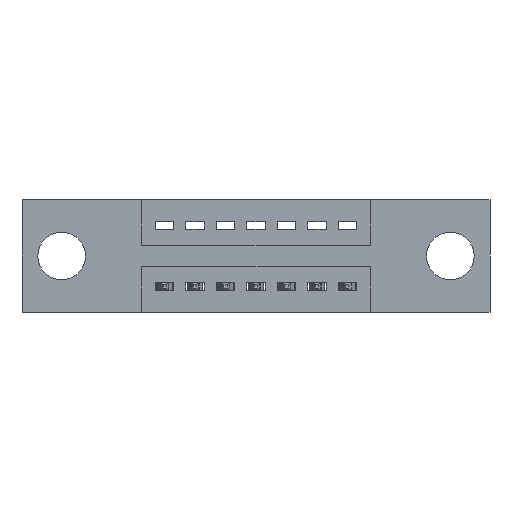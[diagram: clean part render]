
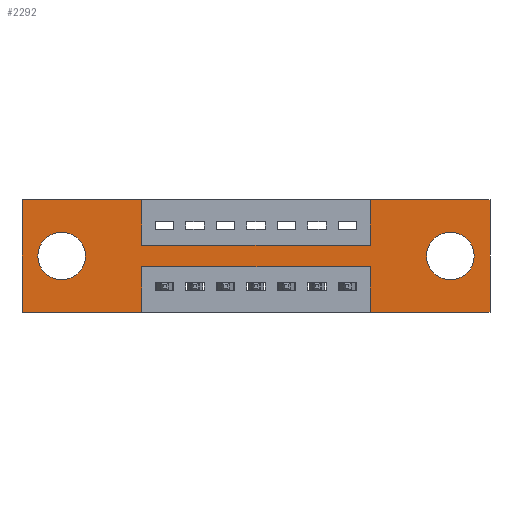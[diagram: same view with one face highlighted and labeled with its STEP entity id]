
A CAD part, front view. The second image highlights one B-rep face of the part: STEP entity #2292.
In plain terms, the highlighted planar face has unit normal (0, -1, 0).
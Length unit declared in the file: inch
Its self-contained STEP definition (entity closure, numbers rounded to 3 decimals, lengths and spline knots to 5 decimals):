
#102 = VERTEX_POINT ( 'NONE', #5162 ) ;
#122 = VERTEX_POINT ( 'NONE', #610 ) ;
#315 = CARTESIAN_POINT ( 'NONE',  ( 1.535, 0., -0.37 ) ) ;
#375 = DIRECTION ( 'NONE',  ( 0., 0., -1. ) ) ;
#422 = PLANE ( 'NONE',  #8379 ) ;
#440 = CARTESIAN_POINT ( 'NONE',  ( 0., 0., -0.37 ) ) ;
#477 = EDGE_CURVE ( 'NONE', #102, #6593, #5903, .T. ) ;
#610 = CARTESIAN_POINT ( 'NONE',  ( 1.405, 0., -0.107 ) ) ;
#1082 = DIRECTION ( 'NONE',  ( 1., 0., 0. ) ) ;
#1196 = DIRECTION ( 'NONE',  ( 0., 1., 0. ) ) ;
#1206 = DIRECTION ( 'NONE',  ( 0., 1., 0. ) ) ;
#1230 = VERTEX_POINT ( 'NONE', #7979 ) ;
#1262 = CARTESIAN_POINT ( 'NONE',  ( 0.3925, 0., -0.22 ) ) ;
#1273 = EDGE_CURVE ( 'NONE', #1230, #5263, #3168, .T. ) ;
#1364 = AXIS2_PLACEMENT_3D ( 'NONE', #6124, #1196, #6824 ) ;
#1372 = VERTEX_POINT ( 'NONE', #6577 ) ;
#1418 = EDGE_CURVE ( 'NONE', #3065, #1230, #2314, .T. ) ;
#1561 = VECTOR ( 'NONE', #375, 39.37008 ) ;
#1761 = EDGE_CURVE ( 'NONE', #5263, #1372, #2443, .T. ) ;
#1782 = EDGE_LOOP ( 'NONE', ( #3721, #3647 ) ) ;
#1783 = EDGE_LOOP ( 'NONE', ( #6504, #3783, #6387, #6543, #3159, #2726, #2746, #2822, #3049, #3062, #4244, #8692 ) ) ;
#1790 = DIRECTION ( 'NONE',  ( 0., 0., 1. ) ) ;
#1834 = CARTESIAN_POINT ( 'NONE',  ( 1.1425, 0., 0. ) ) ;
#1880 = LINE ( 'NONE', #9685, #5927 ) ;
#1946 = CARTESIAN_POINT ( 'NONE',  ( 0.3925, 0., 0. ) ) ;
#2059 = DIRECTION ( 'NONE',  ( 0., 1., 0. ) ) ;
#2099 = CARTESIAN_POINT ( 'NONE',  ( 1.535, 0., 0. ) ) ;
#2210 = VECTOR ( 'NONE', #1790, 39.37008 ) ;
#2235 = CARTESIAN_POINT ( 'NONE',  ( 0.3925, 0., -0.15 ) ) ;
#2292 = ADVANCED_FACE ( 'NONE', ( #9266, #3973, #3713 ), #422, .T. ) ;
#2296 = CARTESIAN_POINT ( 'NONE',  ( 1.1425, 0., -0.15 ) ) ;
#2314 = LINE ( 'NONE', #6392, #6213 ) ;
#2436 = DIRECTION ( 'NONE',  ( 0., 0., 1. ) ) ;
#2443 = LINE ( 'NONE', #2560, #8125 ) ;
#2470 = EDGE_CURVE ( 'NONE', #9956, #102, #7174, .T. ) ;
#2560 = CARTESIAN_POINT ( 'NONE',  ( 0.3925, 0., -0.37 ) ) ;
#2722 = VERTEX_POINT ( 'NONE', #2984 ) ;
#2726 = ORIENTED_EDGE ( 'NONE', *, *, #7229, .F. ) ;
#2746 = ORIENTED_EDGE ( 'NONE', *, *, #6716, .F. ) ;
#2747 = LINE ( 'NONE', #8290, #8345 ) ;
#2766 = CARTESIAN_POINT ( 'NONE',  ( 0.13, 0., -0.263 ) ) ;
#2822 = ORIENTED_EDGE ( 'NONE', *, *, #4788, .F. ) ;
#2856 = VERTEX_POINT ( 'NONE', #315 ) ;
#2984 = CARTESIAN_POINT ( 'NONE',  ( 1.405, 0., -0.263 ) ) ;
#3037 = DIRECTION ( 'NONE',  ( 0., 0., -1. ) ) ;
#3049 = ORIENTED_EDGE ( 'NONE', *, *, #477, .F. ) ;
#3062 = ORIENTED_EDGE ( 'NONE', *, *, #2470, .F. ) ;
#3065 = VERTEX_POINT ( 'NONE', #9720 ) ;
#3159 = ORIENTED_EDGE ( 'NONE', *, *, #6426, .F. ) ;
#3167 = AXIS2_PLACEMENT_3D ( 'NONE', #7868, #7858, #7857 ) ;
#3168 = LINE ( 'NONE', #1262, #6867 ) ;
#3179 = EDGE_CURVE ( 'NONE', #3762, #6191, #5161, .T. ) ;
#3647 = ORIENTED_EDGE ( 'NONE', *, *, #7994, .T. ) ;
#3669 = DIRECTION ( 'NONE',  ( 0., 0., 1. ) ) ;
#3713 = FACE_OUTER_BOUND ( 'NONE', #1783, .T. ) ;
#3721 = ORIENTED_EDGE ( 'NONE', *, *, #5672, .T. ) ;
#3762 = VERTEX_POINT ( 'NONE', #6745 ) ;
#3780 = LINE ( 'NONE', #5933, #7331 ) ;
#3783 = ORIENTED_EDGE ( 'NONE', *, *, #1273, .F. ) ;
#3863 = ORIENTED_EDGE ( 'NONE', *, *, #5044, .T. ) ;
#3973 = FACE_BOUND ( 'NONE', #5759, .T. ) ;
#3983 = LINE ( 'NONE', #10020, #9273 ) ;
#4071 = CARTESIAN_POINT ( 'NONE',  ( 0., 0., 0. ) ) ;
#4097 = CIRCLE ( 'NONE', #7307, 0.078 ) ;
#4244 = ORIENTED_EDGE ( 'NONE', *, *, #4694, .F. ) ;
#4464 = VERTEX_POINT ( 'NONE', #8415 ) ;
#4472 = LINE ( 'NONE', #9650, #6329 ) ;
#4502 = LINE ( 'NONE', #8551, #2210 ) ;
#4656 = CARTESIAN_POINT ( 'NONE',  ( 0., 0., 0. ) ) ;
#4693 = CIRCLE ( 'NONE', #1364, 0.078 ) ;
#4694 = EDGE_CURVE ( 'NONE', #6055, #9956, #4502, .T. ) ;
#4727 = VERTEX_POINT ( 'NONE', #1834 ) ;
#4788 = EDGE_CURVE ( 'NONE', #6593, #5766, #3780, .T. ) ;
#4862 = VECTOR ( 'NONE', #9049, 39.37008 ) ;
#5044 = EDGE_CURVE ( 'NONE', #6191, #3762, #5594, .T. ) ;
#5161 = CIRCLE ( 'NONE', #3167, 0.078 ) ;
#5162 = CARTESIAN_POINT ( 'NONE',  ( 0.3925, 0., 0. ) ) ;
#5240 = EDGE_CURVE ( 'NONE', #2856, #3065, #1880, .T. ) ;
#5263 = VERTEX_POINT ( 'NONE', #6369 ) ;
#5594 = CIRCLE ( 'NONE', #6901, 0.078 ) ;
#5672 = EDGE_CURVE ( 'NONE', #122, #2722, #4693, .T. ) ;
#5759 = EDGE_LOOP ( 'NONE', ( #7292, #3863 ) ) ;
#5766 = VERTEX_POINT ( 'NONE', #2296 ) ;
#5903 = LINE ( 'NONE', #1946, #1561 ) ;
#5927 = VECTOR ( 'NONE', #8389, 39.37008 ) ;
#5933 = CARTESIAN_POINT ( 'NONE',  ( 0.3925, 0., -0.15 ) ) ;
#6055 = VERTEX_POINT ( 'NONE', #7811 ) ;
#6124 = CARTESIAN_POINT ( 'NONE',  ( 1.405, 0., -0.185 ) ) ;
#6133 = CARTESIAN_POINT ( 'NONE',  ( 0.13, 0., -0.185 ) ) ;
#6191 = VERTEX_POINT ( 'NONE', #2766 ) ;
#6213 = VECTOR ( 'NONE', #3669, 39.37008 ) ;
#6243 = DIRECTION ( 'NONE',  ( -1., 0., 0. ) ) ;
#6329 = VECTOR ( 'NONE', #2436, 39.37008 ) ;
#6369 = CARTESIAN_POINT ( 'NONE',  ( 0.3925, 0., -0.22 ) ) ;
#6387 = ORIENTED_EDGE ( 'NONE', *, *, #1418, .F. ) ;
#6392 = CARTESIAN_POINT ( 'NONE',  ( 1.1425, 0., -0.37 ) ) ;
#6426 = EDGE_CURVE ( 'NONE', #4464, #2856, #6434, .T. ) ;
#6434 = LINE ( 'NONE', #2099, #8041 ) ;
#6504 = ORIENTED_EDGE ( 'NONE', *, *, #1761, .F. ) ;
#6543 = ORIENTED_EDGE ( 'NONE', *, *, #5240, .F. ) ;
#6577 = CARTESIAN_POINT ( 'NONE',  ( 0.3925, 0., -0.37 ) ) ;
#6593 = VERTEX_POINT ( 'NONE', #2235 ) ;
#6638 = DIRECTION ( 'NONE',  ( 1., 0., 0. ) ) ;
#6666 = EDGE_CURVE ( 'NONE', #1372, #6055, #2747, .T. ) ;
#6716 = EDGE_CURVE ( 'NONE', #5766, #4727, #4472, .T. ) ;
#6736 = CARTESIAN_POINT ( 'NONE',  ( 1.405, 0., -0.185 ) ) ;
#6745 = CARTESIAN_POINT ( 'NONE',  ( 0.13, 0., -0.107 ) ) ;
#6824 = DIRECTION ( 'NONE',  ( 0., 0., -1. ) ) ;
#6832 = DIRECTION ( 'NONE',  ( 0., 0., 1. ) ) ;
#6867 = VECTOR ( 'NONE', #6243, 39.37008 ) ;
#6901 = AXIS2_PLACEMENT_3D ( 'NONE', #6133, #1206, #6832 ) ;
#7174 = LINE ( 'NONE', #4071, #4862 ) ;
#7229 = EDGE_CURVE ( 'NONE', #4727, #4464, #3983, .T. ) ;
#7292 = ORIENTED_EDGE ( 'NONE', *, *, #3179, .T. ) ;
#7307 = AXIS2_PLACEMENT_3D ( 'NONE', #6736, #2059, #7418 ) ;
#7331 = VECTOR ( 'NONE', #6638, 39.37008 ) ;
#7418 = DIRECTION ( 'NONE',  ( 0., 0., -1. ) ) ;
#7811 = CARTESIAN_POINT ( 'NONE',  ( 0., 0., -0.37 ) ) ;
#7857 = DIRECTION ( 'NONE',  ( 0., 0., 1. ) ) ;
#7858 = DIRECTION ( 'NONE',  ( 0., 1., 0. ) ) ;
#7868 = CARTESIAN_POINT ( 'NONE',  ( 0.13, 0., -0.185 ) ) ;
#7979 = CARTESIAN_POINT ( 'NONE',  ( 1.1425, 0., -0.22 ) ) ;
#7994 = EDGE_CURVE ( 'NONE', #2722, #122, #4097, .T. ) ;
#8041 = VECTOR ( 'NONE', #3037, 39.37008 ) ;
#8086 = DIRECTION ( 'NONE',  ( 0., 0., -1. ) ) ;
#8102 = DIRECTION ( 'NONE',  ( 0., -1., 0. ) ) ;
#8125 = VECTOR ( 'NONE', #8400, 39.37008 ) ;
#8290 = CARTESIAN_POINT ( 'NONE',  ( 0., 0., -0.37 ) ) ;
#8345 = VECTOR ( 'NONE', #8960, 39.37008 ) ;
#8379 = AXIS2_PLACEMENT_3D ( 'NONE', #440, #8102, #8086 ) ;
#8389 = DIRECTION ( 'NONE',  ( -1., 0., 0. ) ) ;
#8400 = DIRECTION ( 'NONE',  ( 0., 0., -1. ) ) ;
#8415 = CARTESIAN_POINT ( 'NONE',  ( 1.535, 0., 0. ) ) ;
#8551 = CARTESIAN_POINT ( 'NONE',  ( 0., 0., 0. ) ) ;
#8692 = ORIENTED_EDGE ( 'NONE', *, *, #6666, .F. ) ;
#8960 = DIRECTION ( 'NONE',  ( -1., 0., 0. ) ) ;
#9049 = DIRECTION ( 'NONE',  ( 1., 0., 0. ) ) ;
#9266 = FACE_BOUND ( 'NONE', #1782, .T. ) ;
#9273 = VECTOR ( 'NONE', #1082, 39.37008 ) ;
#9650 = CARTESIAN_POINT ( 'NONE',  ( 1.1425, 0., 0. ) ) ;
#9685 = CARTESIAN_POINT ( 'NONE',  ( 0., 0., -0.37 ) ) ;
#9720 = CARTESIAN_POINT ( 'NONE',  ( 1.1425, 0., -0.37 ) ) ;
#9956 = VERTEX_POINT ( 'NONE', #4656 ) ;
#10020 = CARTESIAN_POINT ( 'NONE',  ( 0., 0., 0. ) ) ;
